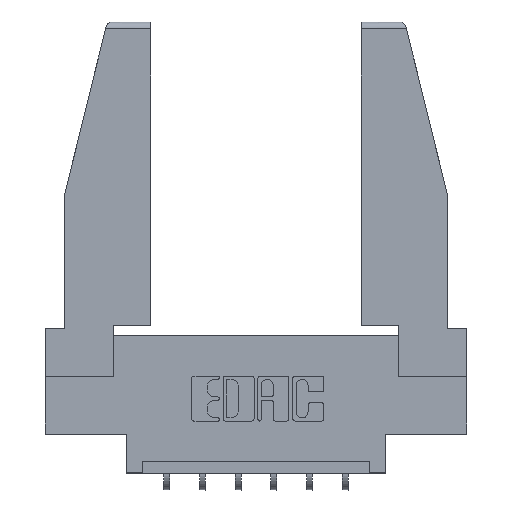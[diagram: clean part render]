
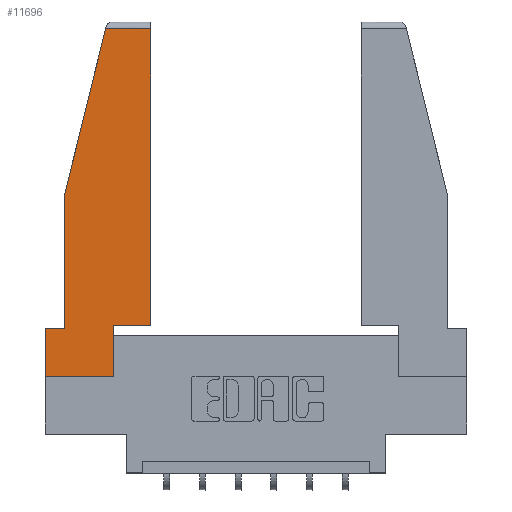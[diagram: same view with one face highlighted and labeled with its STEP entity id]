
A CAD part, top view. The second image highlights one B-rep face of the part: STEP entity #11696.
In plain terms, the highlighted planar face has unit normal (0, 0, 1).
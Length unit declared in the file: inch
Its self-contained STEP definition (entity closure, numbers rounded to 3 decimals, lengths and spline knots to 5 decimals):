
#15 = LINE ( 'NONE', #8172, #2465 ) ;
#71 = CARTESIAN_POINT ( 'NONE',  ( 0.271, 1.55, 0. ) ) ;
#195 = VERTEX_POINT ( 'NONE', #10845 ) ;
#320 = DIRECTION ( 'NONE',  ( -1., 0., 0. ) ) ;
#326 = CARTESIAN_POINT ( 'NONE',  ( 0.086, 0.8, 0. ) ) ;
#341 = VERTEX_POINT ( 'NONE', #5035 ) ;
#366 = CARTESIAN_POINT ( 'NONE',  ( 0., 0., 0. ) ) ;
#706 = ORIENTED_EDGE ( 'NONE', *, *, #895, .T. ) ;
#874 = LINE ( 'NONE', #11109, #7902 ) ;
#895 = EDGE_CURVE ( 'NONE', #2196, #195, #3338, .T. ) ;
#1086 = EDGE_CURVE ( 'NONE', #5073, #4110, #6596, .T. ) ;
#1385 = EDGE_CURVE ( 'NONE', #11410, #5073, #6875, .T. ) ;
#1392 = CARTESIAN_POINT ( 'NONE',  ( 0., 0., 0. ) ) ;
#1607 = VECTOR ( 'NONE', #2306, 39.37008 ) ;
#1663 = CARTESIAN_POINT ( 'NONE',  ( 0.086, 0.8, 0. ) ) ;
#1668 = VERTEX_POINT ( 'NONE', #8752 ) ;
#1993 = LINE ( 'NONE', #9112, #6230 ) ;
#2145 = DIRECTION ( 'NONE',  ( 0., -1., 0. ) ) ;
#2196 = VERTEX_POINT ( 'NONE', #1663 ) ;
#2306 = DIRECTION ( 'NONE',  ( 1., 0., 0. ) ) ;
#2465 = VECTOR ( 'NONE', #4470, 39.37008 ) ;
#2536 = ORIENTED_EDGE ( 'NONE', *, *, #1086, .T. ) ;
#3118 = ORIENTED_EDGE ( 'NONE', *, *, #11121, .T. ) ;
#3277 = ORIENTED_EDGE ( 'NONE', *, *, #4260, .T. ) ;
#3334 = CARTESIAN_POINT ( 'NONE',  ( 0., 0., 0. ) ) ;
#3338 = LINE ( 'NONE', #326, #5315 ) ;
#3349 = ORIENTED_EDGE ( 'NONE', *, *, #1385, .T. ) ;
#3395 = EDGE_CURVE ( 'NONE', #1668, #8915, #1993, .T. ) ;
#3550 = DIRECTION ( 'NONE',  ( 0., -1., 0. ) ) ;
#4011 = FACE_OUTER_BOUND ( 'NONE', #8261, .T. ) ;
#4110 = VERTEX_POINT ( 'NONE', #5871 ) ;
#4257 = ORIENTED_EDGE ( 'NONE', *, *, #8197, .T. ) ;
#4260 = EDGE_CURVE ( 'NONE', #4110, #1668, #7990, .T. ) ;
#4454 = VECTOR ( 'NONE', #3550, 39.37008 ) ;
#4470 = DIRECTION ( 'NONE',  ( 0., 1., 0. ) ) ;
#4752 = EDGE_CURVE ( 'NONE', #195, #11410, #4951, .T. ) ;
#4951 = LINE ( 'NONE', #10770, #11051 ) ;
#5035 = CARTESIAN_POINT ( 'NONE',  ( 0.461, 1.52, 0. ) ) ;
#5073 = VERTEX_POINT ( 'NONE', #3334 ) ;
#5308 = DIRECTION ( 'NONE',  ( 0., 1., 0. ) ) ;
#5315 = VECTOR ( 'NONE', #2145, 39.37008 ) ;
#5697 = DIRECTION ( 'NONE',  ( 1., 0., 0. ) ) ;
#5871 = CARTESIAN_POINT ( 'NONE',  ( 0.297, 0., 0. ) ) ;
#5976 = DIRECTION ( 'NONE',  ( 0., 0., 1. ) ) ;
#6230 = VECTOR ( 'NONE', #5697, 39.37008 ) ;
#6596 = LINE ( 'NONE', #366, #1607 ) ;
#6755 = PLANE ( 'NONE',  #11698 ) ;
#6875 = LINE ( 'NONE', #8996, #4454 ) ;
#7283 = CARTESIAN_POINT ( 'NONE',  ( 0., 0.21, 0. ) ) ;
#7392 = DIRECTION ( 'NONE',  ( -0.239, -0.971, 0. ) ) ;
#7461 = ORIENTED_EDGE ( 'NONE', *, *, #3395, .T. ) ;
#7484 = VERTEX_POINT ( 'NONE', #9975 ) ;
#7902 = VECTOR ( 'NONE', #320, 39.37008 ) ;
#7916 = LINE ( 'NONE', #71, #8054 ) ;
#7990 = LINE ( 'NONE', #10732, #10642 ) ;
#8054 = VECTOR ( 'NONE', #7392, 39.37008 ) ;
#8088 = DIRECTION ( 'NONE',  ( -1., 0., 0. ) ) ;
#8172 = CARTESIAN_POINT ( 'NONE',  ( 0.461, 0.223, 0. ) ) ;
#8197 = EDGE_CURVE ( 'NONE', #341, #7484, #874, .T. ) ;
#8261 = EDGE_LOOP ( 'NONE', ( #3118, #4257, #9053, #706, #8632, #3349, #2536, #3277, #7461 ) ) ;
#8632 = ORIENTED_EDGE ( 'NONE', *, *, #4752, .T. ) ;
#8752 = CARTESIAN_POINT ( 'NONE',  ( 0.297, 0.223, 0. ) ) ;
#8915 = VERTEX_POINT ( 'NONE', #9604 ) ;
#8996 = CARTESIAN_POINT ( 'NONE',  ( 0., 0.21, 0. ) ) ;
#9053 = ORIENTED_EDGE ( 'NONE', *, *, #9809, .T. ) ;
#9112 = CARTESIAN_POINT ( 'NONE',  ( 0.297, 0.223, 0. ) ) ;
#9586 = DIRECTION ( 'NONE',  ( 1., 0., 0. ) ) ;
#9604 = CARTESIAN_POINT ( 'NONE',  ( 0.461, 0.223, 0. ) ) ;
#9809 = EDGE_CURVE ( 'NONE', #7484, #2196, #7916, .T. ) ;
#9975 = CARTESIAN_POINT ( 'NONE',  ( 0.2636, 1.52, 0. ) ) ;
#10642 = VECTOR ( 'NONE', #5308, 39.37008 ) ;
#10732 = CARTESIAN_POINT ( 'NONE',  ( 0.297, 0., 0. ) ) ;
#10770 = CARTESIAN_POINT ( 'NONE',  ( 0., 0.21, 0. ) ) ;
#10845 = CARTESIAN_POINT ( 'NONE',  ( 0.086, 0.21, 0. ) ) ;
#11051 = VECTOR ( 'NONE', #8088, 39.37008 ) ;
#11109 = CARTESIAN_POINT ( 'NONE',  ( 0., 1.52, 0. ) ) ;
#11121 = EDGE_CURVE ( 'NONE', #8915, #341, #15, .T. ) ;
#11410 = VERTEX_POINT ( 'NONE', #7283 ) ;
#11696 = ADVANCED_FACE ( 'NONE', ( #4011 ), #6755, .T. ) ;
#11698 = AXIS2_PLACEMENT_3D ( 'NONE', #1392, #5976, #9586 ) ;
